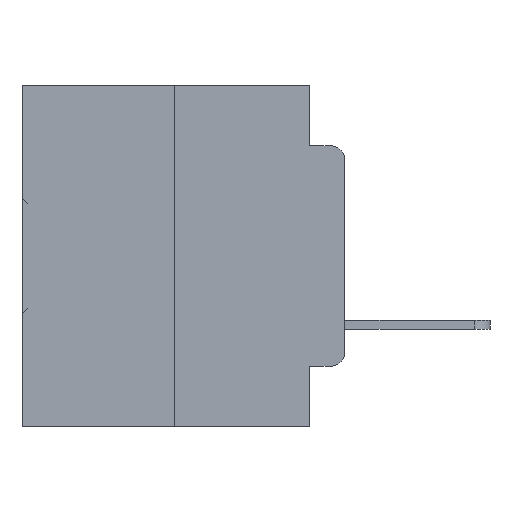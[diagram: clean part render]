
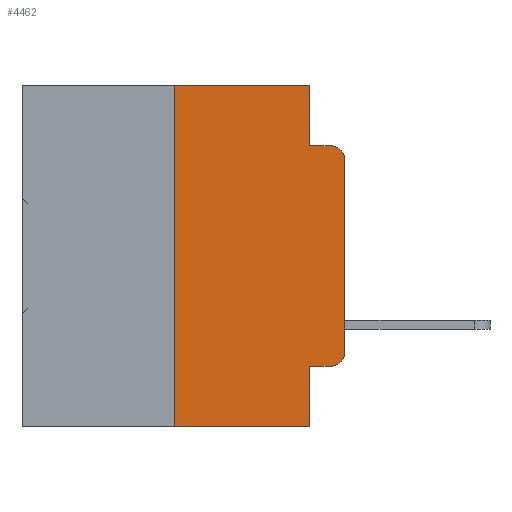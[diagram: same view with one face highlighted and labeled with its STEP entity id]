
A CAD part, left-side view. The second image highlights one B-rep face of the part: STEP entity #4462.
In plain terms, the highlighted planar face has unit normal (-1, 0, 0).
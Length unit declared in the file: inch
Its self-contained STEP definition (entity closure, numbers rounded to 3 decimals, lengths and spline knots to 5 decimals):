
#283 = LINE ( 'NONE', #12443, #10018 ) ;
#317 = VERTEX_POINT ( 'NONE', #30285 ) ;
#318 = DIRECTION ( 'NONE',  ( 0., 0., 1. ) ) ;
#940 = CARTESIAN_POINT ( 'NONE',  ( 0., 0.02, -0.1085 ) ) ;
#1466 = CARTESIAN_POINT ( 'NONE',  ( 0., 0.473, -0.5 ) ) ;
#1488 = VERTEX_POINT ( 'NONE', #3097 ) ;
#2828 = EDGE_CURVE ( 'NONE', #28402, #1488, #23660, .T. ) ;
#3097 = CARTESIAN_POINT ( 'NONE',  ( 0., 0.02, -0.0885 ) ) ;
#3320 = PLANE ( 'NONE',  #6864 ) ;
#3354 = AXIS2_PLACEMENT_3D ( 'NONE', #940, #20492, #3922 ) ;
#3725 = CARTESIAN_POINT ( 'NONE',  ( 0., 0.473, 0. ) ) ;
#3756 = CIRCLE ( 'NONE', #24166, 0.02 ) ;
#3922 = DIRECTION ( 'NONE',  ( 0., 0., -1. ) ) ;
#3943 = VECTOR ( 'NONE', #14497, 39.37008 ) ;
#4462 = ADVANCED_FACE ( 'NONE', ( #33000 ), #3320, .F. ) ;
#4505 = EDGE_LOOP ( 'NONE', ( #33059, #28211, #5372, #19995, #30820, #11244, #29310, #13469, #15990, #8638 ) ) ;
#5065 = EDGE_CURVE ( 'NONE', #27908, #17891, #3756, .T. ) ;
#5148 = CARTESIAN_POINT ( 'NONE',  ( 0., 0.473, 0. ) ) ;
#5372 = ORIENTED_EDGE ( 'NONE', *, *, #2828, .F. ) ;
#6064 = LINE ( 'NONE', #1466, #30611 ) ;
#6781 = DIRECTION ( 'NONE',  ( 0., -1., 0. ) ) ;
#6864 = AXIS2_PLACEMENT_3D ( 'NONE', #5148, #30604, #12586 ) ;
#7086 = EDGE_CURVE ( 'NONE', #21880, #27908, #283, .T. ) ;
#7190 = VECTOR ( 'NONE', #6781, 39.37008 ) ;
#8638 = ORIENTED_EDGE ( 'NONE', *, *, #5065, .T. ) ;
#8765 = EDGE_CURVE ( 'NONE', #25806, #33126, #15495, .T. ) ;
#9816 = CARTESIAN_POINT ( 'NONE',  ( 0., 0.25, -0.5 ) ) ;
#10018 = VECTOR ( 'NONE', #19220, 39.37008 ) ;
#10268 = CARTESIAN_POINT ( 'NONE',  ( 0., 0.051, -0.5 ) ) ;
#11244 = ORIENTED_EDGE ( 'NONE', *, *, #30602, .F. ) ;
#11706 = LINE ( 'NONE', #24729, #3943 ) ;
#12443 = CARTESIAN_POINT ( 'NONE',  ( 0., 0.051, -0.4115 ) ) ;
#12508 = CARTESIAN_POINT ( 'NONE',  ( 0., 0.25, 0. ) ) ;
#12586 = DIRECTION ( 'NONE',  ( 0., 0., -1. ) ) ;
#12959 = CARTESIAN_POINT ( 'NONE',  ( 0., 0.051, 0. ) ) ;
#13469 = ORIENTED_EDGE ( 'NONE', *, *, #24745, .F. ) ;
#14497 = DIRECTION ( 'NONE',  ( 0., 0., -1. ) ) ;
#14908 = EDGE_CURVE ( 'NONE', #17891, #317, #28581, .T. ) ;
#15495 = LINE ( 'NONE', #3725, #7190 ) ;
#15990 = ORIENTED_EDGE ( 'NONE', *, *, #7086, .T. ) ;
#16146 = LINE ( 'NONE', #31580, #28707 ) ;
#17451 = CARTESIAN_POINT ( 'NONE',  ( 0., 0., 0. ) ) ;
#17886 = CIRCLE ( 'NONE', #3354, 0.02 ) ;
#17891 = VERTEX_POINT ( 'NONE', #32134 ) ;
#18164 = EDGE_CURVE ( 'NONE', #21947, #29628, #6064, .T. ) ;
#18165 = VECTOR ( 'NONE', #31391, 39.37008 ) ;
#19220 = DIRECTION ( 'NONE',  ( 0., -1., 0. ) ) ;
#19944 = CARTESIAN_POINT ( 'NONE',  ( 0., 0.02, -0.4115 ) ) ;
#19995 = ORIENTED_EDGE ( 'NONE', *, *, #22827, .F. ) ;
#20492 = DIRECTION ( 'NONE',  ( -1., 0., 0. ) ) ;
#21880 = VERTEX_POINT ( 'NONE', #22795 ) ;
#21947 = VERTEX_POINT ( 'NONE', #9816 ) ;
#22795 = CARTESIAN_POINT ( 'NONE',  ( 0., 0.051, -0.4115 ) ) ;
#22827 = EDGE_CURVE ( 'NONE', #33126, #28402, #24906, .T. ) ;
#23538 = DIRECTION ( 'NONE',  ( 0., -1., 0. ) ) ;
#23660 = LINE ( 'NONE', #25997, #30106 ) ;
#24166 = AXIS2_PLACEMENT_3D ( 'NONE', #34285, #28500, #27850 ) ;
#24729 = CARTESIAN_POINT ( 'NONE',  ( 0., 0.051, 0. ) ) ;
#24745 = EDGE_CURVE ( 'NONE', #21880, #29628, #11706, .T. ) ;
#24906 = LINE ( 'NONE', #26566, #18165 ) ;
#25806 = VERTEX_POINT ( 'NONE', #12508 ) ;
#25997 = CARTESIAN_POINT ( 'NONE',  ( 0., 0.051, -0.0885 ) ) ;
#26566 = CARTESIAN_POINT ( 'NONE',  ( 0., 0.051, 0. ) ) ;
#26963 = DIRECTION ( 'NONE',  ( 0., 0., 1. ) ) ;
#27503 = DIRECTION ( 'NONE',  ( 0., -1., 0. ) ) ;
#27830 = VECTOR ( 'NONE', #318, 39.37008 ) ;
#27850 = DIRECTION ( 'NONE',  ( 0., 0., -1. ) ) ;
#27908 = VERTEX_POINT ( 'NONE', #19944 ) ;
#28051 = EDGE_CURVE ( 'NONE', #317, #1488, #17886, .T. ) ;
#28211 = ORIENTED_EDGE ( 'NONE', *, *, #28051, .T. ) ;
#28402 = VERTEX_POINT ( 'NONE', #33635 ) ;
#28500 = DIRECTION ( 'NONE',  ( -1., 0., 0. ) ) ;
#28581 = LINE ( 'NONE', #17451, #27830 ) ;
#28707 = VECTOR ( 'NONE', #26963, 39.37008 ) ;
#29310 = ORIENTED_EDGE ( 'NONE', *, *, #18164, .T. ) ;
#29628 = VERTEX_POINT ( 'NONE', #10268 ) ;
#30106 = VECTOR ( 'NONE', #27503, 39.37008 ) ;
#30285 = CARTESIAN_POINT ( 'NONE',  ( 0., 0., -0.1085 ) ) ;
#30602 = EDGE_CURVE ( 'NONE', #21947, #25806, #16146, .T. ) ;
#30604 = DIRECTION ( 'NONE',  ( 1., 0., 0. ) ) ;
#30611 = VECTOR ( 'NONE', #23538, 39.37008 ) ;
#30820 = ORIENTED_EDGE ( 'NONE', *, *, #8765, .F. ) ;
#31391 = DIRECTION ( 'NONE',  ( 0., 0., -1. ) ) ;
#31580 = CARTESIAN_POINT ( 'NONE',  ( 0., 0.25, 0. ) ) ;
#32134 = CARTESIAN_POINT ( 'NONE',  ( 0., 0., -0.3915 ) ) ;
#33000 = FACE_OUTER_BOUND ( 'NONE', #4505, .T. ) ;
#33059 = ORIENTED_EDGE ( 'NONE', *, *, #14908, .T. ) ;
#33126 = VERTEX_POINT ( 'NONE', #12959 ) ;
#33635 = CARTESIAN_POINT ( 'NONE',  ( 0., 0.051, -0.0885 ) ) ;
#34285 = CARTESIAN_POINT ( 'NONE',  ( 0., 0.02, -0.3915 ) ) ;
